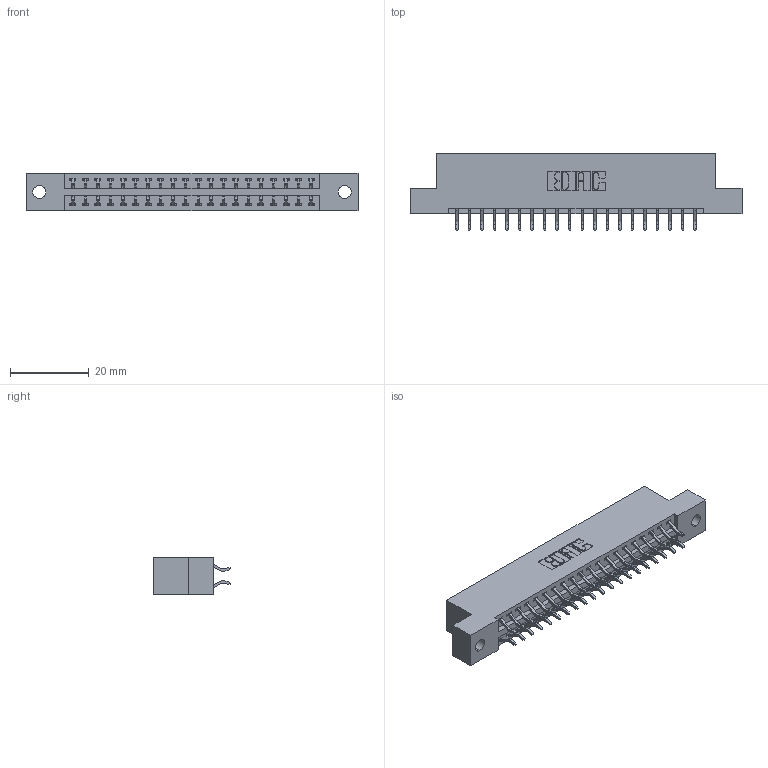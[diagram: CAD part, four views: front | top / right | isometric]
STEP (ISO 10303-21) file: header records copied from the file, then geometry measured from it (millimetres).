
FILE_DESCRIPTION (( 'STEP AP203' ), '1' );
FILE_NAME ('346-040-556-202.STEP', '2018-08-24T10:05:19', ( '' ), ( '' ), 'SwSTEP 2.0', 'SolidWorks 2016', '' );
FILE_SCHEMA (( 'CONFIG_CONTROL_DESIGN' ));
Length unit declared in the file: inch
Products named in the file (3): 346 Part_Flush Mounting Lugs - 0.128 Dia; 345-292-001_556 Tail; 346-040-556-202
Assembly tree (41 placements, depth 2):
  346-040-556-202
    346 Part_Flush Mounting Lugs - 0.128 Dia
    345-292-001_556 Tail  x40
Bounding box: 84.07 x 19.57 x 9.4 mm (x, y, z)
Volume: 7989.1 mm3; surface area: 10329.4 mm2
Topology: 41 solids, 41 shells, 2442 faces, 7249 edges, 4778 vertices
Faces by surface type: plane 1636, cylinder 806
Entity records: 16237 total; most frequent: CARTESIAN_POINT 2720, ORIENTED_EDGE 2642, DIRECTION 2437, EDGE_CURVE 1321, VECTOR 1101, LINE 1101, VERTEX_POINT 878, AXIS2_PLACEMENT_3D 668
